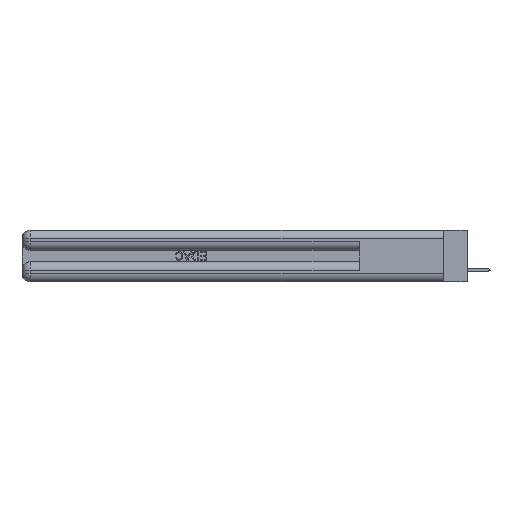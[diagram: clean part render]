
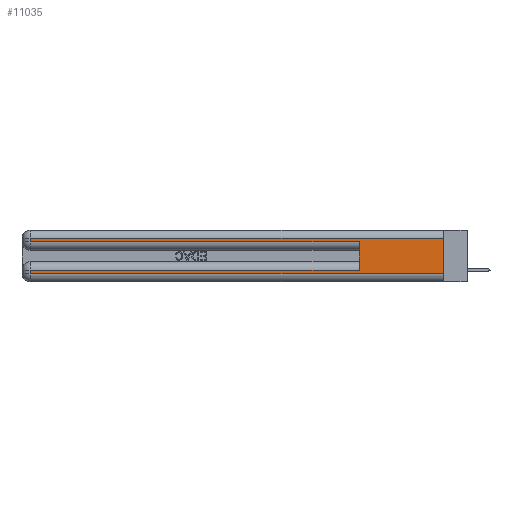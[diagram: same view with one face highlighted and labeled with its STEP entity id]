
A CAD part, left-side view. The second image highlights one B-rep face of the part: STEP entity #11035.
In plain terms, the highlighted planar face has unit normal (-1, 0, 0).
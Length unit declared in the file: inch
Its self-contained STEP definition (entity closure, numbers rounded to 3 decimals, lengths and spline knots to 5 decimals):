
#192 = LINE ( 'NONE', #45445, #44177 ) ;
#391 = LINE ( 'NONE', #40722, #8368 ) ;
#945 = VERTEX_POINT ( 'NONE', #18658 ) ;
#1948 = CARTESIAN_POINT ( 'NONE',  ( 0., 0., 0.06 ) ) ;
#2705 = DIRECTION ( 'NONE',  ( 0., 1., 0. ) ) ;
#2777 = EDGE_CURVE ( 'NONE', #22083, #33914, #16513, .T. ) ;
#3172 = CARTESIAN_POINT ( 'NONE',  ( 0., 2.94, 0.085 ) ) ;
#4549 = ORIENTED_EDGE ( 'NONE', *, *, #7260, .F. ) ;
#4793 = CARTESIAN_POINT ( 'NONE',  ( 0., 2.94, 0.31 ) ) ;
#4804 = EDGE_CURVE ( 'NONE', #5737, #42893, #29817, .T. ) ;
#5737 = VERTEX_POINT ( 'NONE', #17471 ) ;
#5885 = ORIENTED_EDGE ( 'NONE', *, *, #7432, .T. ) ;
#6652 = ORIENTED_EDGE ( 'NONE', *, *, #25927, .T. ) ;
#7260 = EDGE_CURVE ( 'NONE', #22083, #8548, #38741, .T. ) ;
#7432 = EDGE_CURVE ( 'NONE', #945, #42893, #192, .T. ) ;
#7807 = EDGE_CURVE ( 'NONE', #5737, #31667, #31180, .T. ) ;
#8368 = VECTOR ( 'NONE', #8964, 39.37008 ) ;
#8548 = VERTEX_POINT ( 'NONE', #1948 ) ;
#8964 = DIRECTION ( 'NONE',  ( 0., 0., -1. ) ) ;
#9638 = DIRECTION ( 'NONE',  ( 0., 0., -1. ) ) ;
#9813 = ORIENTED_EDGE ( 'NONE', *, *, #20489, .T. ) ;
#9857 = ORIENTED_EDGE ( 'NONE', *, *, #36639, .T. ) ;
#11035 = ADVANCED_FACE ( 'NONE', ( #27124 ), #33741, .F. ) ;
#11174 = DIRECTION ( 'NONE',  ( 0., 0., 1. ) ) ;
#11468 = CARTESIAN_POINT ( 'NONE',  ( 0., 0., 0.31 ) ) ;
#12117 = VECTOR ( 'NONE', #2705, 39.37008 ) ;
#12151 = CARTESIAN_POINT ( 'NONE',  ( 0., 0., 0.37 ) ) ;
#12869 = ORIENTED_EDGE ( 'NONE', *, *, #7807, .T. ) ;
#12947 = CARTESIAN_POINT ( 'NONE',  ( 0., 0.6, 0.145 ) ) ;
#13037 = CARTESIAN_POINT ( 'NONE',  ( 0., 0.6, 0.285 ) ) ;
#13539 = DIRECTION ( 'NONE',  ( 1., 0., 0. ) ) ;
#14597 = LINE ( 'NONE', #25314, #48156 ) ;
#16513 = LINE ( 'NONE', #11468, #47109 ) ;
#17471 = CARTESIAN_POINT ( 'NONE',  ( 0., 0.6, 0.085 ) ) ;
#18658 = CARTESIAN_POINT ( 'NONE',  ( 0., 2.94, 0.285 ) ) ;
#19401 = DIRECTION ( 'NONE',  ( 0., 0., -1. ) ) ;
#20489 = EDGE_CURVE ( 'NONE', #33914, #945, #391, .T. ) ;
#20569 = VECTOR ( 'NONE', #11174, 39.37008 ) ;
#20570 = ORIENTED_EDGE ( 'NONE', *, *, #4804, .F. ) ;
#21359 = DIRECTION ( 'NONE',  ( 0., 0., -1. ) ) ;
#22083 = VERTEX_POINT ( 'NONE', #49057 ) ;
#22292 = CARTESIAN_POINT ( 'NONE',  ( 0., 2.94, 0.06 ) ) ;
#23598 = VERTEX_POINT ( 'NONE', #22292 ) ;
#23794 = EDGE_LOOP ( 'NONE', ( #4549, #24186, #9813, #5885, #20570, #12869, #6652, #9857 ) ) ;
#24186 = ORIENTED_EDGE ( 'NONE', *, *, #2777, .T. ) ;
#25314 = CARTESIAN_POINT ( 'NONE',  ( 0., 2.94, 0.37 ) ) ;
#25927 = EDGE_CURVE ( 'NONE', #31667, #23598, #14597, .T. ) ;
#25983 = CARTESIAN_POINT ( 'NONE',  ( 0., 0., 0.37 ) ) ;
#27124 = FACE_OUTER_BOUND ( 'NONE', #23794, .T. ) ;
#29229 = VECTOR ( 'NONE', #40351, 39.37008 ) ;
#29817 = LINE ( 'NONE', #12947, #20569 ) ;
#30811 = DIRECTION ( 'NONE',  ( 0., 1., 0. ) ) ;
#31180 = LINE ( 'NONE', #37035, #12117 ) ;
#31667 = VERTEX_POINT ( 'NONE', #3172 ) ;
#33741 = PLANE ( 'NONE',  #39465 ) ;
#33914 = VERTEX_POINT ( 'NONE', #4793 ) ;
#36231 = VECTOR ( 'NONE', #19401, 39.37008 ) ;
#36639 = EDGE_CURVE ( 'NONE', #23598, #8548, #40863, .T. ) ;
#37035 = CARTESIAN_POINT ( 'NONE',  ( 0., 0., 0.085 ) ) ;
#38741 = LINE ( 'NONE', #12151, #36231 ) ;
#39465 = AXIS2_PLACEMENT_3D ( 'NONE', #25983, #13539, #21359 ) ;
#40005 = CARTESIAN_POINT ( 'NONE',  ( 0., 0., 0.06 ) ) ;
#40351 = DIRECTION ( 'NONE',  ( 0., -1., 0. ) ) ;
#40722 = CARTESIAN_POINT ( 'NONE',  ( 0., 2.94, 0.37 ) ) ;
#40863 = LINE ( 'NONE', #40005, #29229 ) ;
#42893 = VERTEX_POINT ( 'NONE', #13037 ) ;
#44177 = VECTOR ( 'NONE', #49326, 39.37008 ) ;
#45445 = CARTESIAN_POINT ( 'NONE',  ( 0., 0., 0.285 ) ) ;
#47109 = VECTOR ( 'NONE', #30811, 39.37008 ) ;
#48156 = VECTOR ( 'NONE', #9638, 39.37008 ) ;
#49057 = CARTESIAN_POINT ( 'NONE',  ( 0., 0., 0.31 ) ) ;
#49326 = DIRECTION ( 'NONE',  ( 0., -1., 0. ) ) ;
